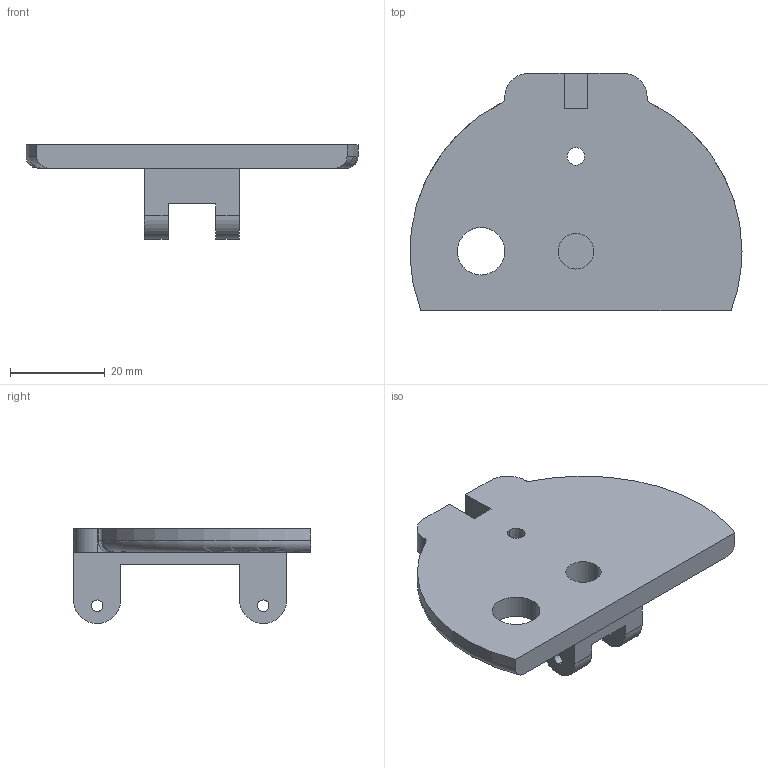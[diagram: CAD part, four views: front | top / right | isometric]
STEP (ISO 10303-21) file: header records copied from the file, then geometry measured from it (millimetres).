
FILE_DESCRIPTION (( 'STEP AP203' ), '1' );
FILE_NAME ('Front_Block.STEP', '2013-11-14T05:07:00', ( '' ), ( '' ), 'SwSTEP 2.0', 'SolidWorks 2013', '' );
FILE_SCHEMA (( 'CONFIG_CONTROL_DESIGN' ));
Length unit declared in the file: millimetre
Products named in the file (1): Front_Block
Bounding box: 69.98 x 50 x 20 mm (x, y, z)
Volume: 17690.9 mm3; surface area: 8898.4 mm2
Topology: 1 solids, 1 shells, 63 faces, 170 edges, 110 vertices
Faces by surface type: cylinder 28, plane 26, cone 4, torus 3, bspline 2
Entity records: 2269 total; most frequent: CARTESIAN_POINT 548, DIRECTION 352, ORIENTED_EDGE 340, EDGE_CURVE 170, AXIS2_PLACEMENT_3D 130, VERTEX_POINT 110, VECTOR 92, LINE 92
